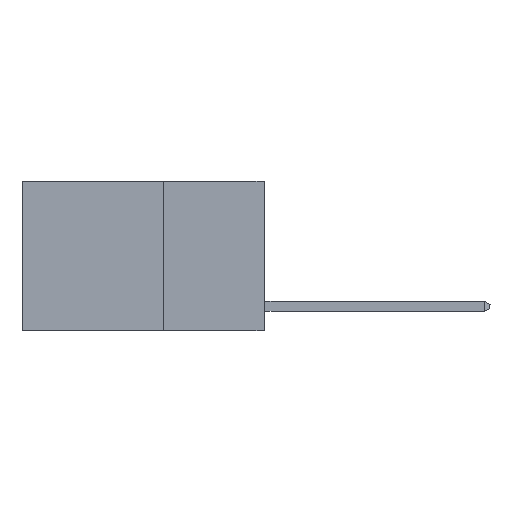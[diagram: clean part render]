
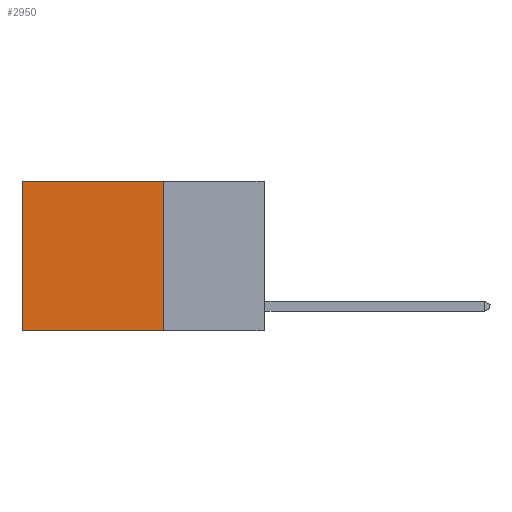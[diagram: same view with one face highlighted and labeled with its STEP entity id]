
A CAD part, left-side view. The second image highlights one B-rep face of the part: STEP entity #2950.
In plain terms, the highlighted planar face has unit normal (-1, 0, 0).
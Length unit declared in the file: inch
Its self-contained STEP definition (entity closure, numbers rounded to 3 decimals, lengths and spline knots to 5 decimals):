
#191 = VECTOR ( 'NONE', #8174, 39.37008 ) ;
#942 = LINE ( 'NONE', #11154, #191 ) ;
#2162 = ORIENTED_EDGE ( 'NONE', *, *, #17654, .T. ) ;
#2528 = EDGE_LOOP ( 'NONE', ( #2162, #4880, #17027, #11405 ) ) ;
#2667 = VERTEX_POINT ( 'NONE', #3640 ) ;
#2755 = AXIS2_PLACEMENT_3D ( 'NONE', #12753, #4285, #5614 ) ;
#2876 = DIRECTION ( 'NONE',  ( 0., 1., 0. ) ) ;
#2950 = ADVANCED_FACE ( 'NONE', ( #5898 ), #6244, .F. ) ;
#3431 = CARTESIAN_POINT ( 'NONE',  ( 0.2625, 0.6, -0.37 ) ) ;
#3640 = CARTESIAN_POINT ( 'NONE',  ( 0.2625, 0.6, 0. ) ) ;
#4285 = DIRECTION ( 'NONE',  ( 1., 0., 0. ) ) ;
#4671 = LINE ( 'NONE', #6191, #11021 ) ;
#4880 = ORIENTED_EDGE ( 'NONE', *, *, #13094, .F. ) ;
#5614 = DIRECTION ( 'NONE',  ( 0., 0., -1. ) ) ;
#5717 = EDGE_CURVE ( 'NONE', #5906, #2667, #13209, .T. ) ;
#5898 = FACE_OUTER_BOUND ( 'NONE', #2528, .T. ) ;
#5906 = VERTEX_POINT ( 'NONE', #6979 ) ;
#6191 = CARTESIAN_POINT ( 'NONE',  ( 0.2625, 0.25, 0. ) ) ;
#6244 = PLANE ( 'NONE',  #2755 ) ;
#6548 = EDGE_CURVE ( 'NONE', #5906, #17881, #4671, .T. ) ;
#6979 = CARTESIAN_POINT ( 'NONE',  ( 0.2625, 0.25, 0. ) ) ;
#7111 = VECTOR ( 'NONE', #2876, 39.37008 ) ;
#8174 = DIRECTION ( 'NONE',  ( 0., 0., -1. ) ) ;
#11021 = VECTOR ( 'NONE', #11526, 39.37008 ) ;
#11154 = CARTESIAN_POINT ( 'NONE',  ( 0.2625, 0.6, 0. ) ) ;
#11405 = ORIENTED_EDGE ( 'NONE', *, *, #5717, .T. ) ;
#11526 = DIRECTION ( 'NONE',  ( 0., 0., -1. ) ) ;
#12688 = DIRECTION ( 'NONE',  ( 0., 1., 0. ) ) ;
#12753 = CARTESIAN_POINT ( 'NONE',  ( 0.2625, 0.25, 0. ) ) ;
#12875 = LINE ( 'NONE', #18324, #18035 ) ;
#13021 = CARTESIAN_POINT ( 'NONE',  ( 0.2625, 0.25, 0. ) ) ;
#13094 = EDGE_CURVE ( 'NONE', #17881, #18372, #12875, .T. ) ;
#13209 = LINE ( 'NONE', #13021, #7111 ) ;
#14371 = CARTESIAN_POINT ( 'NONE',  ( 0.2625, 0.25, -0.37 ) ) ;
#17027 = ORIENTED_EDGE ( 'NONE', *, *, #6548, .F. ) ;
#17654 = EDGE_CURVE ( 'NONE', #2667, #18372, #942, .T. ) ;
#17881 = VERTEX_POINT ( 'NONE', #14371 ) ;
#18035 = VECTOR ( 'NONE', #12688, 39.37008 ) ;
#18324 = CARTESIAN_POINT ( 'NONE',  ( 0.2625, 0.25, -0.37 ) ) ;
#18372 = VERTEX_POINT ( 'NONE', #3431 ) ;
